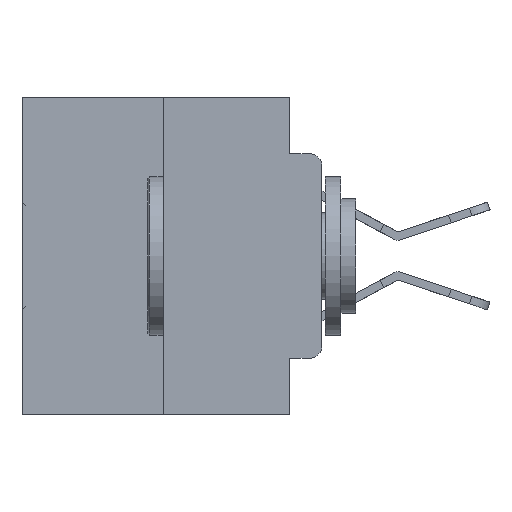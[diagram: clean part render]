
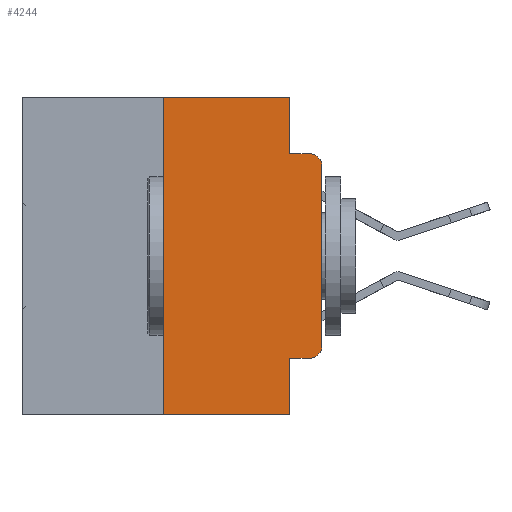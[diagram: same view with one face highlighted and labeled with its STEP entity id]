
A CAD part, left-side view. The second image highlights one B-rep face of the part: STEP entity #4244.
In plain terms, the highlighted planar face has unit normal (-1, 0, 0).
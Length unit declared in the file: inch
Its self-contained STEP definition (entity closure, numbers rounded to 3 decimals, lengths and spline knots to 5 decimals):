
#204 = ORIENTED_EDGE ( 'NONE', *, *, #22463, .T. ) ;
#641 = CIRCLE ( 'NONE', #5090, 0.02 ) ;
#937 = LINE ( 'NONE', #6333, #32399 ) ;
#1029 = DIRECTION ( 'NONE',  ( 0., 0., -1. ) ) ;
#1568 = EDGE_CURVE ( 'NONE', #13680, #5335, #937, .T. ) ;
#1759 = DIRECTION ( 'NONE',  ( 0., -1., 0. ) ) ;
#2650 = ORIENTED_EDGE ( 'NONE', *, *, #28519, .F. ) ;
#2802 = DIRECTION ( 'NONE',  ( 0., 0., -1. ) ) ;
#3031 = ORIENTED_EDGE ( 'NONE', *, *, #5579, .F. ) ;
#3037 = CARTESIAN_POINT ( 'NONE',  ( 0., 0.051, -0.4115 ) ) ;
#3163 = VERTEX_POINT ( 'NONE', #16379 ) ;
#4244 = ADVANCED_FACE ( 'NONE', ( #32819 ), #30211, .F. ) ;
#4457 = DIRECTION ( 'NONE',  ( 0., 0., 1. ) ) ;
#4671 = ORIENTED_EDGE ( 'NONE', *, *, #25571, .F. ) ;
#5090 = AXIS2_PLACEMENT_3D ( 'NONE', #32472, #13516, #32641 ) ;
#5335 = VERTEX_POINT ( 'NONE', #17775 ) ;
#5344 = DIRECTION ( 'NONE',  ( 0., -1., 0. ) ) ;
#5579 = EDGE_CURVE ( 'NONE', #18927, #32729, #31862, .T. ) ;
#6333 = CARTESIAN_POINT ( 'NONE',  ( 0., 0.25, 0. ) ) ;
#6687 = EDGE_CURVE ( 'NONE', #13680, #32729, #8470, .T. ) ;
#6896 = VECTOR ( 'NONE', #20744, 39.37008 ) ;
#7962 = EDGE_CURVE ( 'NONE', #14352, #27484, #641, .T. ) ;
#8470 = LINE ( 'NONE', #13507, #29975 ) ;
#8877 = CARTESIAN_POINT ( 'NONE',  ( 0., 0.02, -0.3915 ) ) ;
#9006 = CARTESIAN_POINT ( 'NONE',  ( 0., 0.473, 0. ) ) ;
#11504 = DIRECTION ( 'NONE',  ( 0., -1., 0. ) ) ;
#12213 = CARTESIAN_POINT ( 'NONE',  ( 0., 0., -0.1085 ) ) ;
#12858 = VECTOR ( 'NONE', #4457, 39.37008 ) ;
#13093 = AXIS2_PLACEMENT_3D ( 'NONE', #8877, #22275, #1029 ) ;
#13507 = CARTESIAN_POINT ( 'NONE',  ( 0., 0.473, -0.5 ) ) ;
#13516 = DIRECTION ( 'NONE',  ( -1., 0., 0. ) ) ;
#13621 = AXIS2_PLACEMENT_3D ( 'NONE', #9006, #19608, #33517 ) ;
#13680 = VERTEX_POINT ( 'NONE', #26046 ) ;
#14262 = CARTESIAN_POINT ( 'NONE',  ( 0., 0.051, 0. ) ) ;
#14352 = VERTEX_POINT ( 'NONE', #12213 ) ;
#14709 = EDGE_CURVE ( 'NONE', #24200, #3163, #21440, .T. ) ;
#14836 = ORIENTED_EDGE ( 'NONE', *, *, #7962, .T. ) ;
#15001 = ORIENTED_EDGE ( 'NONE', *, *, #30831, .T. ) ;
#16379 = CARTESIAN_POINT ( 'NONE',  ( 0., 0., -0.3915 ) ) ;
#17328 = CARTESIAN_POINT ( 'NONE',  ( 0., 0.051, -0.0885 ) ) ;
#17558 = DIRECTION ( 'NONE',  ( 0., 0., -1. ) ) ;
#17761 = LINE ( 'NONE', #30987, #23897 ) ;
#17775 = CARTESIAN_POINT ( 'NONE',  ( 0., 0.25, 0. ) ) ;
#18131 = CARTESIAN_POINT ( 'NONE',  ( 0., 0.051, 0. ) ) ;
#18247 = CARTESIAN_POINT ( 'NONE',  ( 0., 0.02, -0.0885 ) ) ;
#18927 = VERTEX_POINT ( 'NONE', #3037 ) ;
#19441 = ORIENTED_EDGE ( 'NONE', *, *, #21902, .F. ) ;
#19608 = DIRECTION ( 'NONE',  ( 1., 0., 0. ) ) ;
#20451 = VERTEX_POINT ( 'NONE', #17328 ) ;
#20744 = DIRECTION ( 'NONE',  ( 0., -1., 0. ) ) ;
#21440 = CIRCLE ( 'NONE', #13093, 0.02 ) ;
#21902 = EDGE_CURVE ( 'NONE', #24429, #20451, #30266, .T. ) ;
#22168 = DIRECTION ( 'NONE',  ( 0., 0., 1. ) ) ;
#22275 = DIRECTION ( 'NONE',  ( -1., 0., 0. ) ) ;
#22317 = VECTOR ( 'NONE', #11504, 39.37008 ) ;
#22463 = EDGE_CURVE ( 'NONE', #3163, #14352, #26010, .T. ) ;
#22600 = CARTESIAN_POINT ( 'NONE',  ( 0., 0.051, -0.5 ) ) ;
#22704 = CARTESIAN_POINT ( 'NONE',  ( 0., 0.02, -0.4115 ) ) ;
#22820 = VECTOR ( 'NONE', #17558, 39.37008 ) ;
#23685 = CARTESIAN_POINT ( 'NONE',  ( 0., 0.051, -0.4115 ) ) ;
#23897 = VECTOR ( 'NONE', #1759, 39.37008 ) ;
#23971 = ORIENTED_EDGE ( 'NONE', *, *, #6687, .T. ) ;
#23980 = VECTOR ( 'NONE', #2802, 39.37008 ) ;
#24200 = VERTEX_POINT ( 'NONE', #22704 ) ;
#24429 = VERTEX_POINT ( 'NONE', #31389 ) ;
#24719 = LINE ( 'NONE', #25227, #22317 ) ;
#25227 = CARTESIAN_POINT ( 'NONE',  ( 0., 0.051, -0.0885 ) ) ;
#25312 = ORIENTED_EDGE ( 'NONE', *, *, #14709, .T. ) ;
#25571 = EDGE_CURVE ( 'NONE', #5335, #24429, #17761, .T. ) ;
#26010 = LINE ( 'NONE', #33700, #12858 ) ;
#26046 = CARTESIAN_POINT ( 'NONE',  ( 0., 0.25, -0.5 ) ) ;
#26102 = LINE ( 'NONE', #23685, #6896 ) ;
#26926 = ORIENTED_EDGE ( 'NONE', *, *, #1568, .F. ) ;
#27484 = VERTEX_POINT ( 'NONE', #18247 ) ;
#28519 = EDGE_CURVE ( 'NONE', #20451, #27484, #24719, .T. ) ;
#29975 = VECTOR ( 'NONE', #5344, 39.37008 ) ;
#30211 = PLANE ( 'NONE',  #13621 ) ;
#30266 = LINE ( 'NONE', #14262, #22820 ) ;
#30831 = EDGE_CURVE ( 'NONE', #18927, #24200, #26102, .T. ) ;
#30987 = CARTESIAN_POINT ( 'NONE',  ( 0., 0.473, 0. ) ) ;
#31158 = EDGE_LOOP ( 'NONE', ( #204, #14836, #2650, #19441, #4671, #26926, #23971, #3031, #15001, #25312 ) ) ;
#31389 = CARTESIAN_POINT ( 'NONE',  ( 0., 0.051, 0. ) ) ;
#31862 = LINE ( 'NONE', #18131, #23980 ) ;
#32399 = VECTOR ( 'NONE', #22168, 39.37008 ) ;
#32472 = CARTESIAN_POINT ( 'NONE',  ( 0., 0.02, -0.1085 ) ) ;
#32641 = DIRECTION ( 'NONE',  ( 0., 0., -1. ) ) ;
#32729 = VERTEX_POINT ( 'NONE', #22600 ) ;
#32819 = FACE_OUTER_BOUND ( 'NONE', #31158, .T. ) ;
#33517 = DIRECTION ( 'NONE',  ( 0., 0., -1. ) ) ;
#33700 = CARTESIAN_POINT ( 'NONE',  ( 0., 0., 0. ) ) ;
